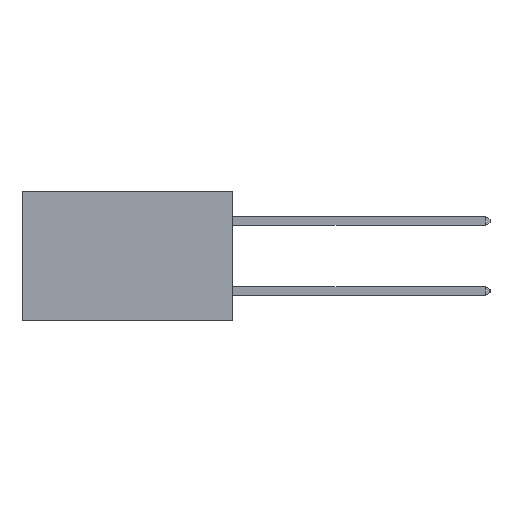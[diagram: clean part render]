
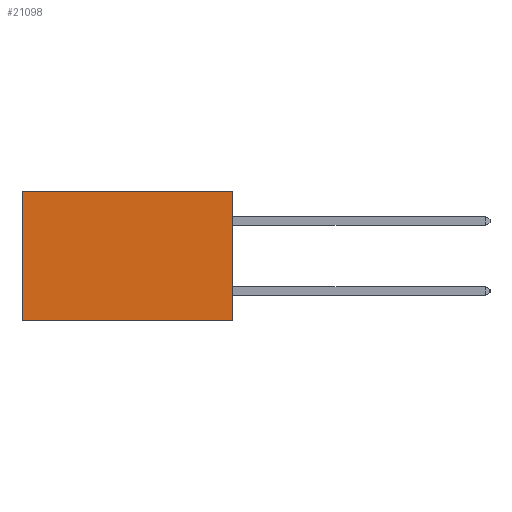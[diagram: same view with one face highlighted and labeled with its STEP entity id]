
A CAD part, left-side view. The second image highlights one B-rep face of the part: STEP entity #21098.
In plain terms, the highlighted planar face has unit normal (-1, 0, 0).
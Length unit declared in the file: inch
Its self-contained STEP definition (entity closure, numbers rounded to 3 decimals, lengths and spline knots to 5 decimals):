
#74 = VERTEX_POINT ( 'NONE', #13476 ) ;
#858 = DIRECTION ( 'NONE',  ( 0., 0., -1. ) ) ;
#965 = EDGE_CURVE ( 'NONE', #16704, #16101, #27975, .T. ) ;
#2880 = CARTESIAN_POINT ( 'NONE',  ( 0.2875, 0., -0.37 ) ) ;
#3271 = DIRECTION ( 'NONE',  ( 0., 1., 0. ) ) ;
#3374 = LINE ( 'NONE', #23040, #10170 ) ;
#3412 = VECTOR ( 'NONE', #28884, 39.37008 ) ;
#6474 = AXIS2_PLACEMENT_3D ( 'NONE', #31326, #17279, #12895 ) ;
#6643 = PLANE ( 'NONE',  #6474 ) ;
#6914 = VECTOR ( 'NONE', #3271, 39.37008 ) ;
#7069 = CARTESIAN_POINT ( 'NONE',  ( 0.2875, 0.6, -0.37 ) ) ;
#9241 = CARTESIAN_POINT ( 'NONE',  ( 0.2875, 0., -0.37 ) ) ;
#9560 = ORIENTED_EDGE ( 'NONE', *, *, #30305, .F. ) ;
#10170 = VECTOR ( 'NONE', #858, 39.37008 ) ;
#12895 = DIRECTION ( 'NONE',  ( 0., 0., -1. ) ) ;
#13000 = ORIENTED_EDGE ( 'NONE', *, *, #965, .F. ) ;
#13189 = LINE ( 'NONE', #31927, #3412 ) ;
#13476 = CARTESIAN_POINT ( 'NONE',  ( 0.2875, 0.6, 0. ) ) ;
#16101 = VERTEX_POINT ( 'NONE', #2880 ) ;
#16704 = VERTEX_POINT ( 'NONE', #17633 ) ;
#17279 = DIRECTION ( 'NONE',  ( 1., 0., 0. ) ) ;
#17633 = CARTESIAN_POINT ( 'NONE',  ( 0.2875, 0., 0. ) ) ;
#20201 = ORIENTED_EDGE ( 'NONE', *, *, #32472, .T. ) ;
#21098 = ADVANCED_FACE ( 'NONE', ( #28265 ), #6643, .F. ) ;
#23040 = CARTESIAN_POINT ( 'NONE',  ( 0.2875, 0.6, 0. ) ) ;
#23098 = VERTEX_POINT ( 'NONE', #7069 ) ;
#24557 = DIRECTION ( 'NONE',  ( 0., 0., -1. ) ) ;
#24898 = CARTESIAN_POINT ( 'NONE',  ( 0.2875, 0., 0. ) ) ;
#25116 = ORIENTED_EDGE ( 'NONE', *, *, #30441, .T. ) ;
#27975 = LINE ( 'NONE', #24898, #35003 ) ;
#28265 = FACE_OUTER_BOUND ( 'NONE', #29173, .T. ) ;
#28884 = DIRECTION ( 'NONE',  ( 0., 1., 0. ) ) ;
#29173 = EDGE_LOOP ( 'NONE', ( #20201, #9560, #13000, #25116 ) ) ;
#30305 = EDGE_CURVE ( 'NONE', #16101, #23098, #33925, .T. ) ;
#30441 = EDGE_CURVE ( 'NONE', #16704, #74, #13189, .T. ) ;
#31326 = CARTESIAN_POINT ( 'NONE',  ( 0.2875, 0., 0. ) ) ;
#31927 = CARTESIAN_POINT ( 'NONE',  ( 0.2875, 0., 0. ) ) ;
#32472 = EDGE_CURVE ( 'NONE', #74, #23098, #3374, .T. ) ;
#33925 = LINE ( 'NONE', #9241, #6914 ) ;
#35003 = VECTOR ( 'NONE', #24557, 39.37008 ) ;
